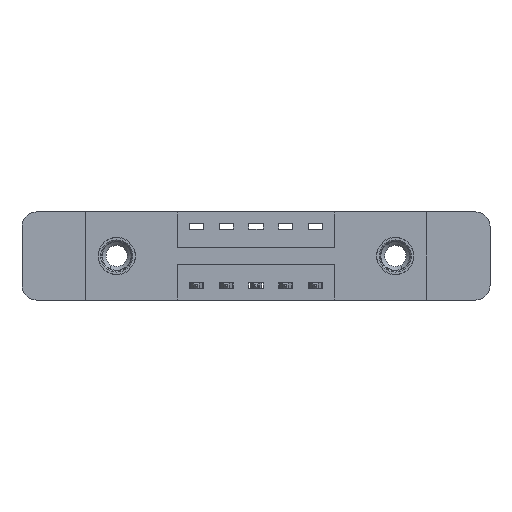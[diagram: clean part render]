
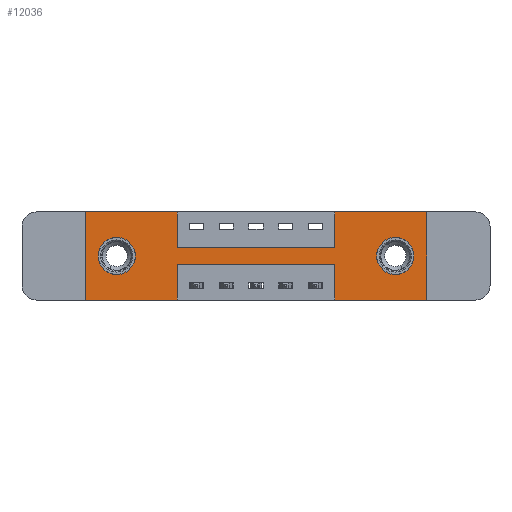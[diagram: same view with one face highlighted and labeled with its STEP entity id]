
A CAD part, front view. The second image highlights one B-rep face of the part: STEP entity #12036.
In plain terms, the highlighted planar face has unit normal (0, -1, 0).
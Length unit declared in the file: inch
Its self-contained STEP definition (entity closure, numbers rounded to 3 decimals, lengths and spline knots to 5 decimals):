
#41 = CARTESIAN_POINT ( 'NONE',  ( 1.3025, 0., -0.185 ) ) ;
#75 = DIRECTION ( 'NONE',  ( 1., 0., 0. ) ) ;
#104 = DIRECTION ( 'NONE',  ( 0., 0., -1. ) ) ;
#139 = VECTOR ( 'NONE', #4760, 39.37008 ) ;
#225 = ORIENTED_EDGE ( 'NONE', *, *, #10628, .F. ) ;
#264 = VECTOR ( 'NONE', #4245, 39.37008 ) ;
#273 = EDGE_LOOP ( 'NONE', ( #1076, #7362 ) ) ;
#295 = LINE ( 'NONE', #369, #139 ) ;
#369 = CARTESIAN_POINT ( 'NONE',  ( 0., 0., 0. ) ) ;
#422 = AXIS2_PLACEMENT_3D ( 'NONE', #10174, #450, #9132 ) ;
#450 = DIRECTION ( 'NONE',  ( 0., 1., 0. ) ) ;
#529 = VECTOR ( 'NONE', #8773, 39.37008 ) ;
#721 = LINE ( 'NONE', #13407, #3774 ) ;
#1076 = ORIENTED_EDGE ( 'NONE', *, *, #10643, .T. ) ;
#1124 = LINE ( 'NONE', #8432, #4817 ) ;
#1413 = DIRECTION ( 'NONE',  ( 0., 0., 1. ) ) ;
#1542 = LINE ( 'NONE', #8910, #3731 ) ;
#1835 = DIRECTION ( 'NONE',  ( 0., -1., 0. ) ) ;
#1978 = CIRCLE ( 'NONE', #422, 0.078 ) ;
#2097 = DIRECTION ( 'NONE',  ( -1., 0., 0. ) ) ;
#2166 = VERTEX_POINT ( 'NONE', #4372 ) ;
#2240 = CARTESIAN_POINT ( 'NONE',  ( 1.0475, 0., -0.15 ) ) ;
#2365 = CIRCLE ( 'NONE', #5700, 0.078 ) ;
#2409 = VERTEX_POINT ( 'NONE', #11394 ) ;
#2579 = EDGE_CURVE ( 'NONE', #11619, #3795, #1542, .T. ) ;
#2586 = VERTEX_POINT ( 'NONE', #9044 ) ;
#2965 = ORIENTED_EDGE ( 'NONE', *, *, #12226, .F. ) ;
#3120 = EDGE_CURVE ( 'NONE', #12942, #12517, #11291, .T. ) ;
#3258 = EDGE_CURVE ( 'NONE', #6014, #11324, #13718, .T. ) ;
#3450 = CARTESIAN_POINT ( 'NONE',  ( 0., 0., 0. ) ) ;
#3639 = CARTESIAN_POINT ( 'NONE',  ( 1.0475, 0., -0.22 ) ) ;
#3653 = VERTEX_POINT ( 'NONE', #12710 ) ;
#3661 = CARTESIAN_POINT ( 'NONE',  ( 1.435, 0., -0.37 ) ) ;
#3731 = VECTOR ( 'NONE', #6961, 39.37008 ) ;
#3774 = VECTOR ( 'NONE', #9331, 39.37008 ) ;
#3795 = VERTEX_POINT ( 'NONE', #12993 ) ;
#4095 = EDGE_CURVE ( 'NONE', #12517, #3653, #8287, .T. ) ;
#4121 = VECTOR ( 'NONE', #12851, 39.37008 ) ;
#4145 = CARTESIAN_POINT ( 'NONE',  ( 0., 0., -0.37 ) ) ;
#4159 = DIRECTION ( 'NONE',  ( 0., 1., 0. ) ) ;
#4245 = DIRECTION ( 'NONE',  ( -1., 0., 0. ) ) ;
#4338 = CARTESIAN_POINT ( 'NONE',  ( 0., 0., 0. ) ) ;
#4372 = CARTESIAN_POINT ( 'NONE',  ( 0., 0., -0.37 ) ) ;
#4601 = ORIENTED_EDGE ( 'NONE', *, *, #4095, .F. ) ;
#4610 = VERTEX_POINT ( 'NONE', #10809 ) ;
#4652 = VERTEX_POINT ( 'NONE', #9747 ) ;
#4666 = EDGE_CURVE ( 'NONE', #9224, #11619, #11877, .T. ) ;
#4760 = DIRECTION ( 'NONE',  ( 0., 0., 1. ) ) ;
#4817 = VECTOR ( 'NONE', #2097, 39.37008 ) ;
#4832 = CARTESIAN_POINT ( 'NONE',  ( 0.1325, 0., -0.185 ) ) ;
#5102 = VECTOR ( 'NONE', #10917, 39.37008 ) ;
#5118 = FACE_BOUND ( 'NONE', #9651, .T. ) ;
#5349 = ORIENTED_EDGE ( 'NONE', *, *, #9054, .T. ) ;
#5370 = ORIENTED_EDGE ( 'NONE', *, *, #7528, .T. ) ;
#5411 = DIRECTION ( 'NONE',  ( 0., 1., 0. ) ) ;
#5676 = ORIENTED_EDGE ( 'NONE', *, *, #7617, .F. ) ;
#5700 = AXIS2_PLACEMENT_3D ( 'NONE', #4832, #9886, #1413 ) ;
#5844 = ORIENTED_EDGE ( 'NONE', *, *, #8845, .F. ) ;
#6014 = VERTEX_POINT ( 'NONE', #3661 ) ;
#6104 = ORIENTED_EDGE ( 'NONE', *, *, #3120, .F. ) ;
#6390 = CIRCLE ( 'NONE', #7503, 0.078 ) ;
#6510 = DIRECTION ( 'NONE',  ( 0., 0., 1. ) ) ;
#6643 = LINE ( 'NONE', #3450, #11397 ) ;
#6904 = ORIENTED_EDGE ( 'NONE', *, *, #7472, .F. ) ;
#6961 = DIRECTION ( 'NONE',  ( 0., 0., -1. ) ) ;
#7039 = EDGE_CURVE ( 'NONE', #4652, #11495, #12310, .T. ) ;
#7128 = DIRECTION ( 'NONE',  ( 0., 0., -1. ) ) ;
#7186 = VERTEX_POINT ( 'NONE', #9002 ) ;
#7278 = DIRECTION ( 'NONE',  ( 0., 0., 1. ) ) ;
#7331 = CARTESIAN_POINT ( 'NONE',  ( 1.0475, 0., 0. ) ) ;
#7362 = ORIENTED_EDGE ( 'NONE', *, *, #7039, .T. ) ;
#7472 = EDGE_CURVE ( 'NONE', #2166, #7186, #295, .T. ) ;
#7503 = AXIS2_PLACEMENT_3D ( 'NONE', #8385, #4159, #7278 ) ;
#7528 = EDGE_CURVE ( 'NONE', #2409, #2586, #2365, .T. ) ;
#7617 = EDGE_CURVE ( 'NONE', #3795, #2166, #1124, .T. ) ;
#7740 = CARTESIAN_POINT ( 'NONE',  ( 0.3875, 0., 0. ) ) ;
#7821 = CARTESIAN_POINT ( 'NONE',  ( 1.435, 0., 0. ) ) ;
#7851 = ORIENTED_EDGE ( 'NONE', *, *, #10759, .F. ) ;
#7909 = CARTESIAN_POINT ( 'NONE',  ( 1.3025, 0., -0.107 ) ) ;
#8170 = PLANE ( 'NONE',  #8318 ) ;
#8194 = CARTESIAN_POINT ( 'NONE',  ( 1.0475, 0., 0. ) ) ;
#8287 = LINE ( 'NONE', #4338, #12367 ) ;
#8318 = AXIS2_PLACEMENT_3D ( 'NONE', #4145, #1835, #7128 ) ;
#8385 = CARTESIAN_POINT ( 'NONE',  ( 0.1325, 0., -0.185 ) ) ;
#8432 = CARTESIAN_POINT ( 'NONE',  ( 0., 0., -0.37 ) ) ;
#8515 = CARTESIAN_POINT ( 'NONE',  ( 0.3875, 0., -0.22 ) ) ;
#8681 = CARTESIAN_POINT ( 'NONE',  ( 1.0475, 0., -0.37 ) ) ;
#8773 = DIRECTION ( 'NONE',  ( -1., 0., 0. ) ) ;
#8814 = ORIENTED_EDGE ( 'NONE', *, *, #2579, .F. ) ;
#8845 = EDGE_CURVE ( 'NONE', #11324, #9224, #13014, .T. ) ;
#8870 = DIRECTION ( 'NONE',  ( 1., 0., 0. ) ) ;
#8910 = CARTESIAN_POINT ( 'NONE',  ( 0.3875, 0., -0.37 ) ) ;
#9002 = CARTESIAN_POINT ( 'NONE',  ( 0., 0., 0. ) ) ;
#9044 = CARTESIAN_POINT ( 'NONE',  ( 0.1325, 0., -0.263 ) ) ;
#9054 = EDGE_CURVE ( 'NONE', #2586, #2409, #6390, .T. ) ;
#9132 = DIRECTION ( 'NONE',  ( 0., 0., -1. ) ) ;
#9223 = AXIS2_PLACEMENT_3D ( 'NONE', #41, #5411, #104 ) ;
#9224 = VERTEX_POINT ( 'NONE', #3639 ) ;
#9331 = DIRECTION ( 'NONE',  ( 0., 0., -1. ) ) ;
#9333 = FACE_OUTER_BOUND ( 'NONE', #9618, .T. ) ;
#9423 = CARTESIAN_POINT ( 'NONE',  ( 0., 0., -0.37 ) ) ;
#9618 = EDGE_LOOP ( 'NONE', ( #8814, #12021, #5844, #10386, #225, #4601, #6104, #2965, #7851, #12925, #6904, #5676 ) ) ;
#9651 = EDGE_LOOP ( 'NONE', ( #5370, #5349 ) ) ;
#9747 = CARTESIAN_POINT ( 'NONE',  ( 1.3025, 0., -0.263 ) ) ;
#9886 = DIRECTION ( 'NONE',  ( 0., 1., 0. ) ) ;
#10174 = CARTESIAN_POINT ( 'NONE',  ( 1.3025, 0., -0.185 ) ) ;
#10261 = DIRECTION ( 'NONE',  ( 0., 0., 1. ) ) ;
#10386 = ORIENTED_EDGE ( 'NONE', *, *, #3258, .F. ) ;
#10628 = EDGE_CURVE ( 'NONE', #3653, #6014, #12024, .T. ) ;
#10643 = EDGE_CURVE ( 'NONE', #11495, #4652, #1978, .T. ) ;
#10665 = CARTESIAN_POINT ( 'NONE',  ( 1.0475, 0., -0.37 ) ) ;
#10698 = LINE ( 'NONE', #12778, #4121 ) ;
#10759 = EDGE_CURVE ( 'NONE', #11153, #4610, #721, .T. ) ;
#10809 = CARTESIAN_POINT ( 'NONE',  ( 0.3875, 0., -0.15 ) ) ;
#10839 = CARTESIAN_POINT ( 'NONE',  ( 0.3875, 0., -0.22 ) ) ;
#10917 = DIRECTION ( 'NONE',  ( 0., 0., -1. ) ) ;
#11153 = VERTEX_POINT ( 'NONE', #7740 ) ;
#11291 = LINE ( 'NONE', #8194, #12441 ) ;
#11324 = VERTEX_POINT ( 'NONE', #8681 ) ;
#11394 = CARTESIAN_POINT ( 'NONE',  ( 0.1325, 0., -0.107 ) ) ;
#11397 = VECTOR ( 'NONE', #8870, 39.37008 ) ;
#11495 = VERTEX_POINT ( 'NONE', #7909 ) ;
#11619 = VERTEX_POINT ( 'NONE', #8515 ) ;
#11680 = VECTOR ( 'NONE', #6510, 39.37008 ) ;
#11821 = EDGE_CURVE ( 'NONE', #7186, #11153, #6643, .T. ) ;
#11877 = LINE ( 'NONE', #10839, #529 ) ;
#12021 = ORIENTED_EDGE ( 'NONE', *, *, #4666, .F. ) ;
#12024 = LINE ( 'NONE', #7821, #5102 ) ;
#12036 = ADVANCED_FACE ( 'NONE', ( #12377, #5118, #9333 ), #8170, .T. ) ;
#12226 = EDGE_CURVE ( 'NONE', #4610, #12942, #10698, .T. ) ;
#12310 = CIRCLE ( 'NONE', #9223, 0.078 ) ;
#12367 = VECTOR ( 'NONE', #75, 39.37008 ) ;
#12377 = FACE_BOUND ( 'NONE', #273, .T. ) ;
#12441 = VECTOR ( 'NONE', #10261, 39.37008 ) ;
#12517 = VERTEX_POINT ( 'NONE', #7331 ) ;
#12710 = CARTESIAN_POINT ( 'NONE',  ( 1.435, 0., 0. ) ) ;
#12778 = CARTESIAN_POINT ( 'NONE',  ( 0.3875, 0., -0.15 ) ) ;
#12851 = DIRECTION ( 'NONE',  ( 1., 0., 0. ) ) ;
#12925 = ORIENTED_EDGE ( 'NONE', *, *, #11821, .F. ) ;
#12942 = VERTEX_POINT ( 'NONE', #2240 ) ;
#12993 = CARTESIAN_POINT ( 'NONE',  ( 0.3875, 0., -0.37 ) ) ;
#13014 = LINE ( 'NONE', #10665, #11680 ) ;
#13407 = CARTESIAN_POINT ( 'NONE',  ( 0.3875, 0., 0. ) ) ;
#13718 = LINE ( 'NONE', #9423, #264 ) ;
